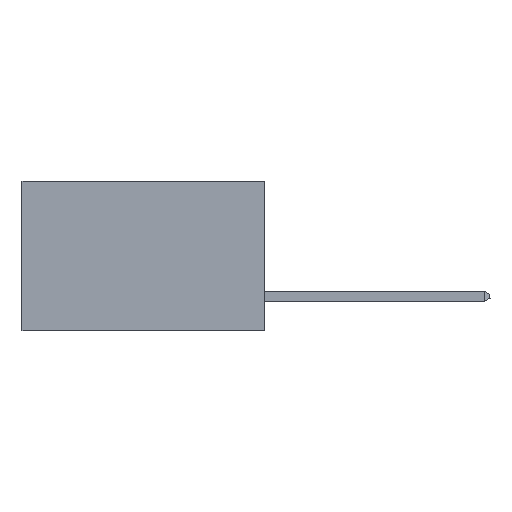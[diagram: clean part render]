
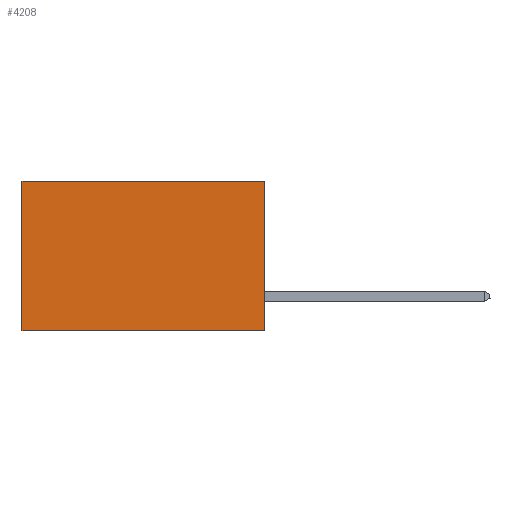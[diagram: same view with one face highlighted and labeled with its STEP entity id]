
A CAD part, left-side view. The second image highlights one B-rep face of the part: STEP entity #4208.
In plain terms, the highlighted planar face has unit normal (-1, 0, 0).
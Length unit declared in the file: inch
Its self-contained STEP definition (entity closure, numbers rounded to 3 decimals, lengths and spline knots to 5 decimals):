
#84 = CARTESIAN_POINT ( 'NONE',  ( 0.2615, 0., 0. ) ) ;
#1062 = DIRECTION ( 'NONE',  ( 0., 0., -1. ) ) ;
#1189 = EDGE_CURVE ( 'NONE', #4310, #8833, #10289, .T. ) ;
#1245 = CARTESIAN_POINT ( 'NONE',  ( 0.2615, 0., -0.37 ) ) ;
#1703 = ORIENTED_EDGE ( 'NONE', *, *, #9637, .T. ) ;
#1971 = ORIENTED_EDGE ( 'NONE', *, *, #1189, .T. ) ;
#2236 = DIRECTION ( 'NONE',  ( 1., 0., 0. ) ) ;
#2293 = LINE ( 'NONE', #9694, #10445 ) ;
#2671 = EDGE_CURVE ( 'NONE', #8874, #8833, #4186, .T. ) ;
#3285 = PLANE ( 'NONE',  #6437 ) ;
#3713 = CARTESIAN_POINT ( 'NONE',  ( 0.2615, 0.6, -0.37 ) ) ;
#3826 = FACE_OUTER_BOUND ( 'NONE', #5431, .T. ) ;
#3898 = DIRECTION ( 'NONE',  ( 0., 0., -1. ) ) ;
#4186 = LINE ( 'NONE', #12710, #13414 ) ;
#4208 = ADVANCED_FACE ( 'NONE', ( #3826 ), #3285, .F. ) ;
#4254 = ORIENTED_EDGE ( 'NONE', *, *, #8238, .F. ) ;
#4310 = VERTEX_POINT ( 'NONE', #12062 ) ;
#4724 = LINE ( 'NONE', #84, #5411 ) ;
#5192 = DIRECTION ( 'NONE',  ( 0., 1., 0. ) ) ;
#5411 = VECTOR ( 'NONE', #11836, 39.37008 ) ;
#5431 = EDGE_LOOP ( 'NONE', ( #1971, #11212, #4254, #1703 ) ) ;
#6437 = AXIS2_PLACEMENT_3D ( 'NONE', #1245, #2236, #9600 ) ;
#8238 = EDGE_CURVE ( 'NONE', #10044, #8874, #2293, .T. ) ;
#8833 = VERTEX_POINT ( 'NONE', #11642 ) ;
#8874 = VERTEX_POINT ( 'NONE', #10609 ) ;
#9061 = CARTESIAN_POINT ( 'NONE',  ( 0.2615, 0., 0. ) ) ;
#9600 = DIRECTION ( 'NONE',  ( 0., 0., -1. ) ) ;
#9637 = EDGE_CURVE ( 'NONE', #10044, #4310, #4724, .T. ) ;
#9694 = CARTESIAN_POINT ( 'NONE',  ( 0.2615, 0., -0.37 ) ) ;
#10044 = VERTEX_POINT ( 'NONE', #9061 ) ;
#10289 = LINE ( 'NONE', #3713, #13153 ) ;
#10445 = VECTOR ( 'NONE', #1062, 39.37008 ) ;
#10609 = CARTESIAN_POINT ( 'NONE',  ( 0.2615, 0., -0.37 ) ) ;
#11212 = ORIENTED_EDGE ( 'NONE', *, *, #2671, .F. ) ;
#11642 = CARTESIAN_POINT ( 'NONE',  ( 0.2615, 0.6, -0.37 ) ) ;
#11836 = DIRECTION ( 'NONE',  ( 0., 1., 0. ) ) ;
#12062 = CARTESIAN_POINT ( 'NONE',  ( 0.2615, 0.6, 0. ) ) ;
#12710 = CARTESIAN_POINT ( 'NONE',  ( 0.2615, 0., -0.37 ) ) ;
#13153 = VECTOR ( 'NONE', #3898, 39.37008 ) ;
#13414 = VECTOR ( 'NONE', #5192, 39.37008 ) ;
